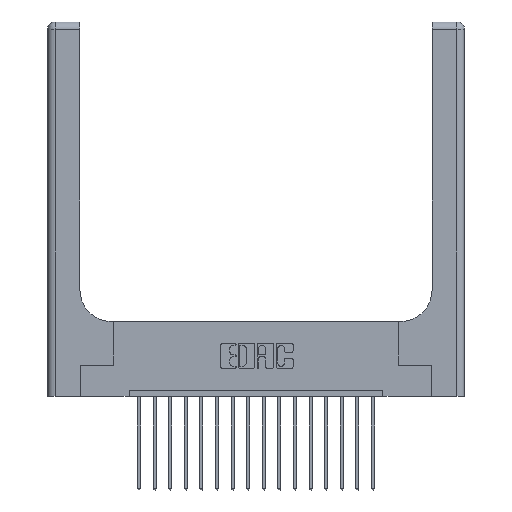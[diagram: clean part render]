
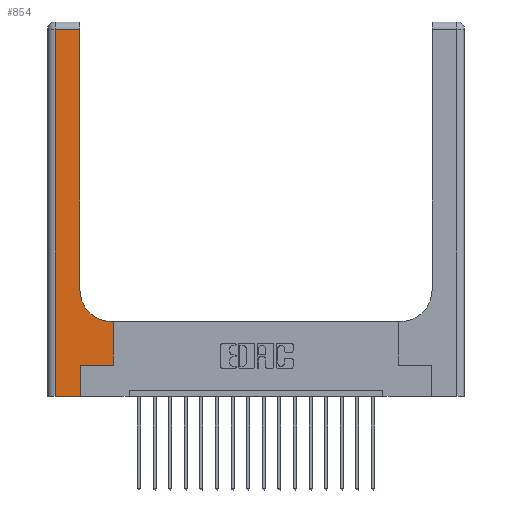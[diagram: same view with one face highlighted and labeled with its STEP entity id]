
A CAD part, top view. The second image highlights one B-rep face of the part: STEP entity #854.
In plain terms, the highlighted planar face has unit normal (0, 0, 1).
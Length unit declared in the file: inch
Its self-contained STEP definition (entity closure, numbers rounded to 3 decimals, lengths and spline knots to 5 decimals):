
#228 = LINE ( 'NONE', #6951, #3622 ) ;
#717 = ORIENTED_EDGE ( 'NONE', *, *, #11398, .T. ) ;
#854 = ADVANCED_FACE ( 'NONE', ( #10481 ), #14027, .F. ) ;
#1100 = CARTESIAN_POINT ( 'NONE',  ( 0.51, 0.6, 0.37 ) ) ;
#1447 = ORIENTED_EDGE ( 'NONE', *, *, #12529, .T. ) ;
#1808 = CARTESIAN_POINT ( 'NONE',  ( 0.26, 0.85, 0.37 ) ) ;
#2182 = VERTEX_POINT ( 'NONE', #12818 ) ;
#2276 = DIRECTION ( 'NONE',  ( 1., 0., 0. ) ) ;
#2291 = EDGE_CURVE ( 'NONE', #9551, #2870, #15176, .T. ) ;
#2462 = ORIENTED_EDGE ( 'NONE', *, *, #8001, .T. ) ;
#2515 = VERTEX_POINT ( 'NONE', #10327 ) ;
#2870 = VERTEX_POINT ( 'NONE', #8606 ) ;
#2929 = ORIENTED_EDGE ( 'NONE', *, *, #15351, .T. ) ;
#3097 = ORIENTED_EDGE ( 'NONE', *, *, #4712, .T. ) ;
#3214 = DIRECTION ( 'NONE',  ( -1., 0., 0. ) ) ;
#3327 = VECTOR ( 'NONE', #18493, 39.37008 ) ;
#3425 = AXIS2_PLACEMENT_3D ( 'NONE', #5247, #15389, #11168 ) ;
#3451 = AXIS2_PLACEMENT_3D ( 'NONE', #16015, #14640, #10438 ) ;
#3622 = VECTOR ( 'NONE', #18129, 39.37008 ) ;
#4346 = CARTESIAN_POINT ( 'NONE',  ( 0.06, 2.94, 0.37 ) ) ;
#4517 = EDGE_CURVE ( 'NONE', #10626, #2515, #4737, .T. ) ;
#4712 = EDGE_CURVE ( 'NONE', #11186, #14143, #13321, .T. ) ;
#4737 = LINE ( 'NONE', #8361, #10805 ) ;
#5219 = DIRECTION ( 'NONE',  ( 0., 1., 0. ) ) ;
#5247 = CARTESIAN_POINT ( 'NONE',  ( 0., 3., 0.37 ) ) ;
#5488 = VECTOR ( 'NONE', #2276, 39.37008 ) ;
#5494 = VERTEX_POINT ( 'NONE', #1808 ) ;
#5664 = CARTESIAN_POINT ( 'NONE',  ( 0.265, 0.25, 0.37 ) ) ;
#6951 = CARTESIAN_POINT ( 'NONE',  ( 0., 0., 0.37 ) ) ;
#6967 = ORIENTED_EDGE ( 'NONE', *, *, #18263, .T. ) ;
#6988 = VECTOR ( 'NONE', #12026, 39.37008 ) ;
#7017 = ORIENTED_EDGE ( 'NONE', *, *, #16916, .T. ) ;
#8001 = EDGE_CURVE ( 'NONE', #2182, #9551, #9576, .T. ) ;
#8012 = VECTOR ( 'NONE', #3214, 39.37008 ) ;
#8361 = CARTESIAN_POINT ( 'NONE',  ( 0.528, 0.25, 0.37 ) ) ;
#8362 = CARTESIAN_POINT ( 'NONE',  ( 0.528, 0.25, 0.37 ) ) ;
#8606 = CARTESIAN_POINT ( 'NONE',  ( 0.06, 0., 0.37 ) ) ;
#9395 = EDGE_LOOP ( 'NONE', ( #1447, #2462, #18513, #717, #3097, #6967, #18270, #2929, #7017 ) ) ;
#9551 = VERTEX_POINT ( 'NONE', #4346 ) ;
#9576 = LINE ( 'NONE', #17567, #8012 ) ;
#9652 = LINE ( 'NONE', #18210, #13520 ) ;
#9778 = VECTOR ( 'NONE', #14709, 39.37008 ) ;
#10089 = CARTESIAN_POINT ( 'NONE',  ( 0.06, 3., 0.37 ) ) ;
#10327 = CARTESIAN_POINT ( 'NONE',  ( 0.528, 0.6, 0.37 ) ) ;
#10438 = DIRECTION ( 'NONE',  ( 1., 0., 0. ) ) ;
#10481 = FACE_OUTER_BOUND ( 'NONE', #9395, .T. ) ;
#10626 = VERTEX_POINT ( 'NONE', #8362 ) ;
#10805 = VECTOR ( 'NONE', #15731, 39.37008 ) ;
#10855 = CARTESIAN_POINT ( 'NONE',  ( 0.265, 0.25, 0.37 ) ) ;
#11168 = DIRECTION ( 'NONE',  ( -1., 0., 0. ) ) ;
#11186 = VERTEX_POINT ( 'NONE', #17770 ) ;
#11398 = EDGE_CURVE ( 'NONE', #2870, #11186, #228, .T. ) ;
#11528 = VERTEX_POINT ( 'NONE', #1100 ) ;
#11613 = CARTESIAN_POINT ( 'NONE',  ( 0.26, 0.6, 0.37 ) ) ;
#11918 = LINE ( 'NONE', #11613, #3327 ) ;
#12026 = DIRECTION ( 'NONE',  ( 0., 1., 0. ) ) ;
#12529 = EDGE_CURVE ( 'NONE', #5494, #2182, #9652, .T. ) ;
#12818 = CARTESIAN_POINT ( 'NONE',  ( 0.26, 2.94, 0.37 ) ) ;
#13321 = LINE ( 'NONE', #17897, #6988 ) ;
#13520 = VECTOR ( 'NONE', #5219, 39.37008 ) ;
#14027 = PLANE ( 'NONE',  #3425 ) ;
#14143 = VERTEX_POINT ( 'NONE', #5664 ) ;
#14640 = DIRECTION ( 'NONE',  ( 0., 0., -1. ) ) ;
#14709 = DIRECTION ( 'NONE',  ( 0., -1., 0. ) ) ;
#15176 = LINE ( 'NONE', #10089, #9778 ) ;
#15180 = LINE ( 'NONE', #10855, #5488 ) ;
#15351 = EDGE_CURVE ( 'NONE', #2515, #11528, #11918, .T. ) ;
#15389 = DIRECTION ( 'NONE',  ( 0., 0., -1. ) ) ;
#15474 = CIRCLE ( 'NONE', #3451, 0.25 ) ;
#15731 = DIRECTION ( 'NONE',  ( 0., 1., 0. ) ) ;
#16015 = CARTESIAN_POINT ( 'NONE',  ( 0.51, 0.85, 0.37 ) ) ;
#16916 = EDGE_CURVE ( 'NONE', #11528, #5494, #15474, .T. ) ;
#17567 = CARTESIAN_POINT ( 'NONE',  ( 0., 2.94, 0.37 ) ) ;
#17770 = CARTESIAN_POINT ( 'NONE',  ( 0.265, 0., 0.37 ) ) ;
#17897 = CARTESIAN_POINT ( 'NONE',  ( 0.265, 0., 0.37 ) ) ;
#18129 = DIRECTION ( 'NONE',  ( 1., 0., 0. ) ) ;
#18210 = CARTESIAN_POINT ( 'NONE',  ( 0.26, 3., 0.37 ) ) ;
#18263 = EDGE_CURVE ( 'NONE', #14143, #10626, #15180, .T. ) ;
#18270 = ORIENTED_EDGE ( 'NONE', *, *, #4517, .T. ) ;
#18493 = DIRECTION ( 'NONE',  ( -1., 0., 0. ) ) ;
#18513 = ORIENTED_EDGE ( 'NONE', *, *, #2291, .T. ) ;
